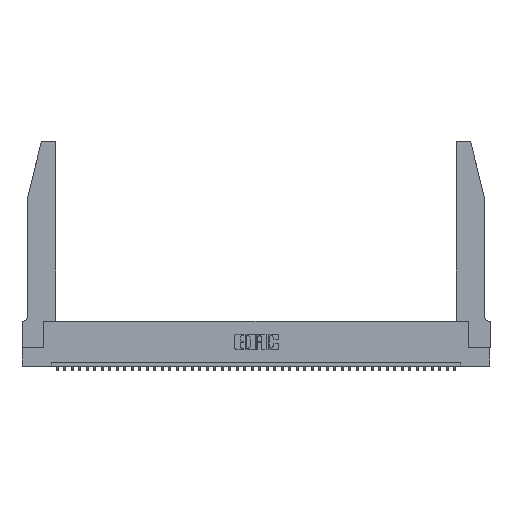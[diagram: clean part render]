
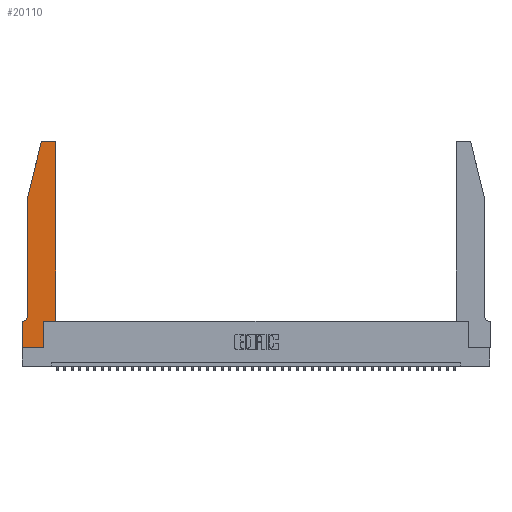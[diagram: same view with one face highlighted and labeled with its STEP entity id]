
A CAD part, top view. The second image highlights one B-rep face of the part: STEP entity #20110.
In plain terms, the highlighted planar face has unit normal (0, 0, 1).
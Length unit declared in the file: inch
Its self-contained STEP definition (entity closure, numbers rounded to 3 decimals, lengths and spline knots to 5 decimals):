
#232 = AXIS2_PLACEMENT_3D ( 'NONE', #16874, #17012, #33905 ) ;
#345 = DIRECTION ( 'NONE',  ( -1., 0., 0. ) ) ;
#540 = CARTESIAN_POINT ( 'NONE',  ( 0.2865, 0.35, 0.37 ) ) ;
#943 = CARTESIAN_POINT ( 'NONE',  ( 0.0755, 2., 0.37 ) ) ;
#1222 = CIRCLE ( 'NONE', #2391, 0.07 ) ;
#1826 = ORIENTED_EDGE ( 'NONE', *, *, #7983, .T. ) ;
#2391 = AXIS2_PLACEMENT_3D ( 'NONE', #11330, #21705, #8233 ) ;
#2472 = CARTESIAN_POINT ( 'NONE',  ( 0.4505, 0.35, 0.37 ) ) ;
#2769 = CARTESIAN_POINT ( 'NONE',  ( 0.4505, 0.35, 0.37 ) ) ;
#2972 = AXIS2_PLACEMENT_3D ( 'NONE', #16682, #16383, #36667 ) ;
#3398 = EDGE_CURVE ( 'NONE', #28711, #40919, #26165, .T. ) ;
#3890 = VECTOR ( 'NONE', #22633, 39.37008 ) ;
#4142 = ORIENTED_EDGE ( 'NONE', *, *, #32979, .T. ) ;
#4544 = CARTESIAN_POINT ( 'NONE',  ( 0.4505, 2.72, 0.37 ) ) ;
#5710 = LINE ( 'NONE', #25062, #26347 ) ;
#6271 = CARTESIAN_POINT ( 'NONE',  ( 0.2865, 0., 0.37 ) ) ;
#6282 = ORIENTED_EDGE ( 'NONE', *, *, #17105, .T. ) ;
#6311 = VECTOR ( 'NONE', #12364, 39.37008 ) ;
#6642 = LINE ( 'NONE', #33942, #17753 ) ;
#7519 = CARTESIAN_POINT ( 'NONE',  ( 0.0755, 0.42, 0.37 ) ) ;
#7983 = EDGE_CURVE ( 'NONE', #24898, #22384, #10701, .T. ) ;
#8233 = DIRECTION ( 'NONE',  ( -1., 0., 0. ) ) ;
#8352 = CIRCLE ( 'NONE', #26903, 0.03 ) ;
#9117 = VERTEX_POINT ( 'NONE', #6271 ) ;
#10089 = CARTESIAN_POINT ( 'NONE',  ( 0.4205, 2.72, 0.37 ) ) ;
#10701 = CIRCLE ( 'NONE', #232, 0.03 ) ;
#10891 = DIRECTION ( 'NONE',  ( -0.239, -0.971, 0. ) ) ;
#10906 = CARTESIAN_POINT ( 'NONE',  ( 0., 0.35, 0.37 ) ) ;
#11330 = CARTESIAN_POINT ( 'NONE',  ( 0.0055, 0.42, 0.37 ) ) ;
#12221 = DIRECTION ( 'NONE',  ( 1., 0., 0. ) ) ;
#12364 = DIRECTION ( 'NONE',  ( -1., 0., 0. ) ) ;
#12494 = CARTESIAN_POINT ( 'NONE',  ( 0.284, 2.75, 0.37 ) ) ;
#13046 = DIRECTION ( 'NONE',  ( 1., 0., 0. ) ) ;
#13290 = DIRECTION ( 'NONE',  ( 0., 1., 0. ) ) ;
#14170 = DIRECTION ( 'NONE',  ( 0., -1., 0. ) ) ;
#14655 = CARTESIAN_POINT ( 'NONE',  ( 0.4205, 2.75, 0.37 ) ) ;
#14696 = VECTOR ( 'NONE', #345, 39.37008 ) ;
#15026 = CARTESIAN_POINT ( 'NONE',  ( 0.25487, 2.72718, 0.37 ) ) ;
#16046 = ORIENTED_EDGE ( 'NONE', *, *, #23875, .T. ) ;
#16201 = VERTEX_POINT ( 'NONE', #42720 ) ;
#16383 = DIRECTION ( 'NONE',  ( 0., 0., 1. ) ) ;
#16410 = EDGE_CURVE ( 'NONE', #30102, #24898, #29077, .T. ) ;
#16574 = DIRECTION ( 'NONE',  ( 0., 0., 1. ) ) ;
#16682 = CARTESIAN_POINT ( 'NONE',  ( 0., 0.35, 0.37 ) ) ;
#16874 = CARTESIAN_POINT ( 'NONE',  ( 0.284, 2.72, 0.37 ) ) ;
#17012 = DIRECTION ( 'NONE',  ( 0., 0., 1. ) ) ;
#17105 = EDGE_CURVE ( 'NONE', #22384, #41667, #5710, .T. ) ;
#17753 = VECTOR ( 'NONE', #37319, 39.37008 ) ;
#20110 = ADVANCED_FACE ( 'NONE', ( #29281 ), #23076, .T. ) ;
#20699 = EDGE_CURVE ( 'NONE', #16201, #9117, #26067, .T. ) ;
#21705 = DIRECTION ( 'NONE',  ( 0., 0., -1. ) ) ;
#22384 = VERTEX_POINT ( 'NONE', #15026 ) ;
#22633 = DIRECTION ( 'NONE',  ( 1., 0., 0. ) ) ;
#23076 = PLANE ( 'NONE',  #2972 ) ;
#23875 = EDGE_CURVE ( 'NONE', #41316, #30102, #8352, .T. ) ;
#24898 = VERTEX_POINT ( 'NONE', #12494 ) ;
#25062 = CARTESIAN_POINT ( 'NONE',  ( 0.0755, 2., 0.37 ) ) ;
#25157 = EDGE_CURVE ( 'NONE', #40919, #41316, #6642, .T. ) ;
#25932 = EDGE_LOOP ( 'NONE', ( #35509, #1826, #6282, #4142, #29098, #26144, #38854, #35008, #27242, #31352, #26263, #16046 ) ) ;
#25958 = CARTESIAN_POINT ( 'NONE',  ( 0., 0., 0.37 ) ) ;
#26067 = LINE ( 'NONE', #25958, #43527 ) ;
#26144 = ORIENTED_EDGE ( 'NONE', *, *, #32777, .T. ) ;
#26165 = LINE ( 'NONE', #2769, #3890 ) ;
#26263 = ORIENTED_EDGE ( 'NONE', *, *, #25157, .T. ) ;
#26347 = VECTOR ( 'NONE', #10891, 39.37008 ) ;
#26903 = AXIS2_PLACEMENT_3D ( 'NONE', #10089, #16574, #13046 ) ;
#27242 = ORIENTED_EDGE ( 'NONE', *, *, #31068, .T. ) ;
#28711 = VERTEX_POINT ( 'NONE', #540 ) ;
#28978 = LINE ( 'NONE', #34574, #33255 ) ;
#29077 = LINE ( 'NONE', #39438, #6311 ) ;
#29098 = ORIENTED_EDGE ( 'NONE', *, *, #39665, .T. ) ;
#29281 = FACE_OUTER_BOUND ( 'NONE', #25932, .T. ) ;
#30102 = VERTEX_POINT ( 'NONE', #14655 ) ;
#30451 = CARTESIAN_POINT ( 'NONE',  ( 0.2865, 0.35, 0.37 ) ) ;
#30622 = EDGE_CURVE ( 'NONE', #39538, #16201, #39179, .T. ) ;
#30912 = CARTESIAN_POINT ( 'NONE',  ( 0., 0., 0.37 ) ) ;
#31068 = EDGE_CURVE ( 'NONE', #9117, #28711, #33371, .T. ) ;
#31352 = ORIENTED_EDGE ( 'NONE', *, *, #3398, .T. ) ;
#32777 = EDGE_CURVE ( 'NONE', #36006, #39538, #42730, .T. ) ;
#32979 = EDGE_CURVE ( 'NONE', #41667, #35016, #28978, .T. ) ;
#33255 = VECTOR ( 'NONE', #37653, 39.37008 ) ;
#33371 = LINE ( 'NONE', #30451, #37562 ) ;
#33395 = CARTESIAN_POINT ( 'NONE',  ( 0.0055, 0.35, 0.37 ) ) ;
#33905 = DIRECTION ( 'NONE',  ( 1., 0., 0. ) ) ;
#33942 = CARTESIAN_POINT ( 'NONE',  ( 0.4505, 0.35, 0.37 ) ) ;
#34574 = CARTESIAN_POINT ( 'NONE',  ( 0.0755, 2., 0.37 ) ) ;
#35008 = ORIENTED_EDGE ( 'NONE', *, *, #20699, .T. ) ;
#35016 = VERTEX_POINT ( 'NONE', #7519 ) ;
#35509 = ORIENTED_EDGE ( 'NONE', *, *, #16410, .T. ) ;
#36006 = VERTEX_POINT ( 'NONE', #33395 ) ;
#36202 = CARTESIAN_POINT ( 'NONE',  ( 0.0755, 0.35, 0.37 ) ) ;
#36667 = DIRECTION ( 'NONE',  ( 1., 0., 0. ) ) ;
#37319 = DIRECTION ( 'NONE',  ( 0., 1., 0. ) ) ;
#37562 = VECTOR ( 'NONE', #13290, 39.37008 ) ;
#37653 = DIRECTION ( 'NONE',  ( 0., -1., 0. ) ) ;
#38854 = ORIENTED_EDGE ( 'NONE', *, *, #30622, .T. ) ;
#39179 = LINE ( 'NONE', #30912, #40269 ) ;
#39438 = CARTESIAN_POINT ( 'NONE',  ( 0.2605, 2.75, 0.37 ) ) ;
#39538 = VERTEX_POINT ( 'NONE', #10906 ) ;
#39665 = EDGE_CURVE ( 'NONE', #35016, #36006, #1222, .T. ) ;
#40269 = VECTOR ( 'NONE', #14170, 39.37008 ) ;
#40919 = VERTEX_POINT ( 'NONE', #2472 ) ;
#41316 = VERTEX_POINT ( 'NONE', #4544 ) ;
#41667 = VERTEX_POINT ( 'NONE', #943 ) ;
#42720 = CARTESIAN_POINT ( 'NONE',  ( 0., 0., 0.37 ) ) ;
#42730 = LINE ( 'NONE', #36202, #14696 ) ;
#43527 = VECTOR ( 'NONE', #12221, 39.37008 ) ;
